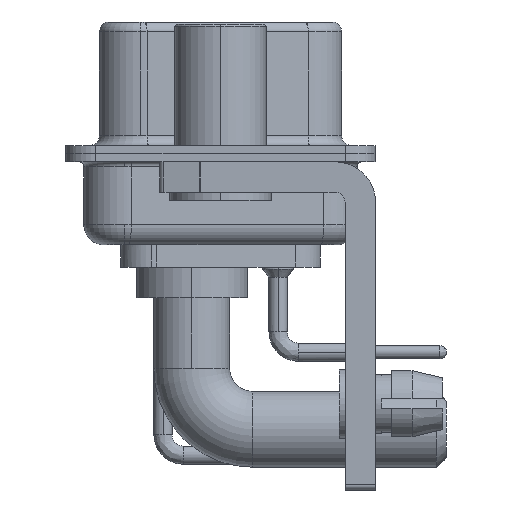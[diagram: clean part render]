
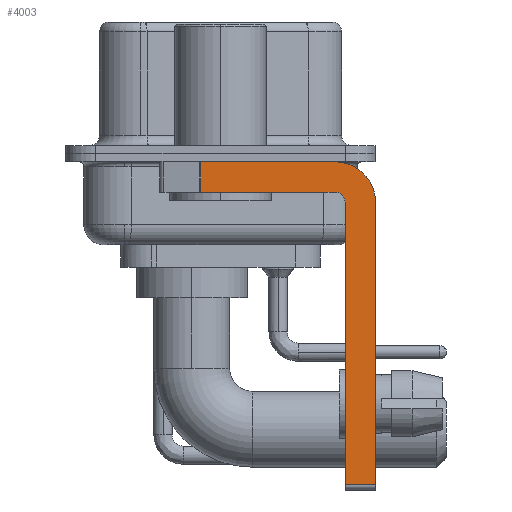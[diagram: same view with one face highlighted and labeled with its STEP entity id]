
A CAD part, left-side view. The second image highlights one B-rep face of the part: STEP entity #4003.
In plain terms, the highlighted planar face has unit normal (-1, 0, 0).
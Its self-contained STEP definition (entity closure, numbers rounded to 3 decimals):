
#423 = LINE ( 'NONE', #12243, #14978 ) ;
#549 = FACE_OUTER_BOUND ( 'NONE', #20958, .T. ) ;
#2576 = EDGE_CURVE ( 'NONE', #16222, #21800, #28475, .T. ) ;
#2987 = CARTESIAN_POINT ( 'NONE',  ( -2.9, -5.65, -1.9 ) ) ;
#3684 = LINE ( 'NONE', #32785, #27037 ) ;
#4003 = ADVANCED_FACE ( 'NONE', ( #549 ), #21096, .F. ) ;
#4593 = EDGE_CURVE ( 'NONE', #16222, #38015, #37728, .T. ) ;
#4770 = AXIS2_PLACEMENT_3D ( 'NONE', #30765, #25337, #28243 ) ;
#4975 = DIRECTION ( 'NONE',  ( 0., 0., -1. ) ) ;
#6744 = ORIENTED_EDGE ( 'NONE', *, *, #12164, .F. ) ;
#6854 = CARTESIAN_POINT ( 'NONE',  ( -2.9, 0.978, -0.4 ) ) ;
#7265 = EDGE_CURVE ( 'NONE', #18538, #32137, #25524, .T. ) ;
#7823 = ORIENTED_EDGE ( 'NONE', *, *, #12723, .F. ) ;
#7884 = CARTESIAN_POINT ( 'NONE',  ( -2.9, -5.65, -0.4 ) ) ;
#8501 = ORIENTED_EDGE ( 'NONE', *, *, #18876, .F. ) ;
#8982 = VERTEX_POINT ( 'NONE', #7884 ) ;
#9986 = AXIS2_PLACEMENT_3D ( 'NONE', #16967, #23160, #16773 ) ;
#11007 = CARTESIAN_POINT ( 'NONE',  ( -2.9, -5.65, -1.9 ) ) ;
#11969 = EDGE_CURVE ( 'NONE', #8982, #33737, #21740, .T. ) ;
#12164 = EDGE_CURVE ( 'NONE', #15820, #32137, #17723, .T. ) ;
#12243 = CARTESIAN_POINT ( 'NONE',  ( -2.9, -7.65, -2.4 ) ) ;
#12286 = DIRECTION ( 'NONE',  ( 0., 1., 0. ) ) ;
#12366 = DIRECTION ( 'NONE',  ( 1., 0., 0. ) ) ;
#12378 = CARTESIAN_POINT ( 'NONE',  ( -2.9, -6.15, -2.4 ) ) ;
#12723 = EDGE_CURVE ( 'NONE', #33737, #21800, #423, .T. ) ;
#13889 = CARTESIAN_POINT ( 'NONE',  ( -2.9, 0.978, -1.9 ) ) ;
#14455 = CARTESIAN_POINT ( 'NONE',  ( -2.9, -6.15, -16.35 ) ) ;
#14978 = VECTOR ( 'NONE', #15355, 1000. ) ;
#15355 = DIRECTION ( 'NONE',  ( 0., 0., -1. ) ) ;
#15589 = ORIENTED_EDGE ( 'NONE', *, *, #4593, .F. ) ;
#15820 = VERTEX_POINT ( 'NONE', #11007 ) ;
#16222 = VERTEX_POINT ( 'NONE', #14455 ) ;
#16579 = DIRECTION ( 'NONE',  ( 0., 0., 1. ) ) ;
#16773 = DIRECTION ( 'NONE',  ( 0., 0., -1. ) ) ;
#16791 = VECTOR ( 'NONE', #12286, 1000. ) ;
#16967 = CARTESIAN_POINT ( 'NONE',  ( -2.9, -5.65, -2.4 ) ) ;
#17723 = LINE ( 'NONE', #2987, #16791 ) ;
#17907 = ORIENTED_EDGE ( 'NONE', *, *, #20643, .F. ) ;
#18186 = CARTESIAN_POINT ( 'NONE',  ( -2.9, -5.65, -2.4 ) ) ;
#18538 = VERTEX_POINT ( 'NONE', #6854 ) ;
#18876 = EDGE_CURVE ( 'NONE', #18538, #8982, #3684, .T. ) ;
#19563 = DIRECTION ( 'NONE',  ( 0., -1., 0. ) ) ;
#19644 = CARTESIAN_POINT ( 'NONE',  ( -2.9, -7.65, -2.4 ) ) ;
#19946 = CARTESIAN_POINT ( 'NONE',  ( -2.9, -5.65, -16.35 ) ) ;
#20643 = EDGE_CURVE ( 'NONE', #38015, #15820, #22080, .T. ) ;
#20958 = EDGE_LOOP ( 'NONE', ( #8501, #30705, #6744, #17907, #15589, #22441, #7823, #34219 ) ) ;
#21096 = PLANE ( 'NONE',  #26711 ) ;
#21740 = CIRCLE ( 'NONE', #9986, 2. ) ;
#21800 = VERTEX_POINT ( 'NONE', #24990 ) ;
#22080 = CIRCLE ( 'NONE', #4770, 0.5 ) ;
#22441 = ORIENTED_EDGE ( 'NONE', *, *, #2576, .T. ) ;
#23035 = VECTOR ( 'NONE', #4975, 1000. ) ;
#23160 = DIRECTION ( 'NONE',  ( 1., 0., 0. ) ) ;
#24266 = VECTOR ( 'NONE', #19563, 1000. ) ;
#24990 = CARTESIAN_POINT ( 'NONE',  ( -2.9, -7.65, -16.35 ) ) ;
#25337 = DIRECTION ( 'NONE',  ( -1., 0., 0. ) ) ;
#25524 = LINE ( 'NONE', #13889, #23035 ) ;
#26350 = DIRECTION ( 'NONE',  ( 0., 0., -1. ) ) ;
#26711 = AXIS2_PLACEMENT_3D ( 'NONE', #18186, #12366, #26350 ) ;
#27037 = VECTOR ( 'NONE', #36093, 1000. ) ;
#28243 = DIRECTION ( 'NONE',  ( 0., 0., 1. ) ) ;
#28475 = LINE ( 'NONE', #19946, #24266 ) ;
#30705 = ORIENTED_EDGE ( 'NONE', *, *, #7265, .T. ) ;
#30765 = CARTESIAN_POINT ( 'NONE',  ( -2.9, -5.65, -2.4 ) ) ;
#32137 = VERTEX_POINT ( 'NONE', #32802 ) ;
#32785 = CARTESIAN_POINT ( 'NONE',  ( -2.9, 3., -0.4 ) ) ;
#32802 = CARTESIAN_POINT ( 'NONE',  ( -2.9, 0.978, -1.9 ) ) ;
#33737 = VERTEX_POINT ( 'NONE', #19644 ) ;
#34219 = ORIENTED_EDGE ( 'NONE', *, *, #11969, .F. ) ;
#34811 = CARTESIAN_POINT ( 'NONE',  ( -2.9, -6.15, -16.6 ) ) ;
#36093 = DIRECTION ( 'NONE',  ( 0., -1., 0. ) ) ;
#37728 = LINE ( 'NONE', #34811, #37939 ) ;
#37939 = VECTOR ( 'NONE', #16579, 1000. ) ;
#38015 = VERTEX_POINT ( 'NONE', #12378 ) ;
